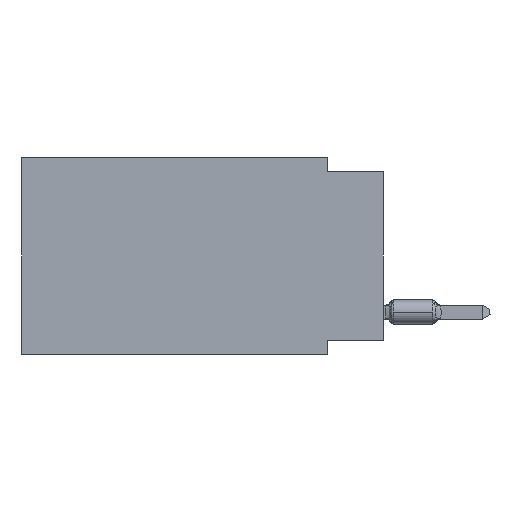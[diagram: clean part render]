
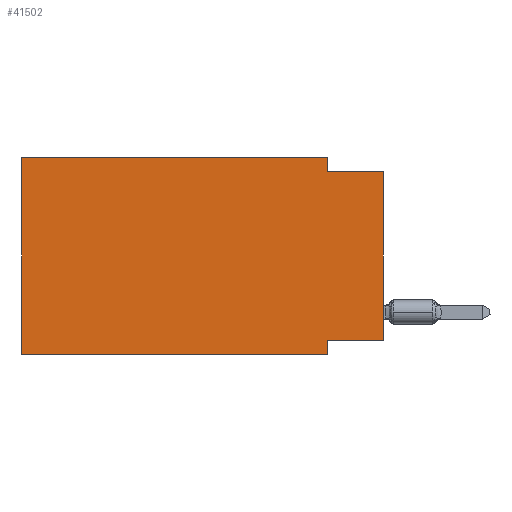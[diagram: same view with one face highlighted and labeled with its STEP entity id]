
A CAD part, left-side view. The second image highlights one B-rep face of the part: STEP entity #41502.
In plain terms, the highlighted planar face has unit normal (-1, 0, 0).
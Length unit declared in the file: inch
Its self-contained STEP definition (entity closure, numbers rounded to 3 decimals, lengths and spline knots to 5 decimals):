
#730 = LINE ( 'NONE', #33870, #26013 ) ;
#1937 = FACE_OUTER_BOUND ( 'NONE', #45939, .T. ) ;
#2708 = ORIENTED_EDGE ( 'NONE', *, *, #36477, .F. ) ;
#2786 = EDGE_CURVE ( 'NONE', #45251, #16510, #2845, .T. ) ;
#2845 = LINE ( 'NONE', #39812, #20690 ) ;
#5706 = DIRECTION ( 'NONE',  ( 0., 0., 1. ) ) ;
#6420 = LINE ( 'NONE', #46501, #44992 ) ;
#8974 = CARTESIAN_POINT ( 'NONE',  ( 0., 0.1, -0.35 ) ) ;
#9756 = ORIENTED_EDGE ( 'NONE', *, *, #10498, .T. ) ;
#9972 = DIRECTION ( 'NONE',  ( 0., -1., 0. ) ) ;
#10498 = EDGE_CURVE ( 'NONE', #33811, #16510, #16093, .T. ) ;
#12027 = DIRECTION ( 'NONE',  ( 0., 0., -1. ) ) ;
#12107 = CARTESIAN_POINT ( 'NONE',  ( 0., 0.645, 0. ) ) ;
#12514 = CARTESIAN_POINT ( 'NONE',  ( 0., 0.645, 0. ) ) ;
#13005 = LINE ( 'NONE', #16838, #44288 ) ;
#13292 = VECTOR ( 'NONE', #22812, 39.37008 ) ;
#15845 = DIRECTION ( 'NONE',  ( 0., -1., 0. ) ) ;
#16093 = LINE ( 'NONE', #41045, #37263 ) ;
#16480 = ORIENTED_EDGE ( 'NONE', *, *, #17004, .F. ) ;
#16510 = VERTEX_POINT ( 'NONE', #8974 ) ;
#16838 = CARTESIAN_POINT ( 'NONE',  ( 0., 0., -0.325 ) ) ;
#16841 = DIRECTION ( 'NONE',  ( 0., 0., -1. ) ) ;
#17004 = EDGE_CURVE ( 'NONE', #26796, #45251, #13005, .T. ) ;
#17196 = CARTESIAN_POINT ( 'NONE',  ( 0., 0., -0.025 ) ) ;
#17506 = DIRECTION ( 'NONE',  ( 0., 0., -1. ) ) ;
#18779 = EDGE_CURVE ( 'NONE', #23331, #19464, #730, .T. ) ;
#19195 = CARTESIAN_POINT ( 'NONE',  ( 0., 0.1, -0.325 ) ) ;
#19464 = VERTEX_POINT ( 'NONE', #34119 ) ;
#20690 = VECTOR ( 'NONE', #17506, 39.37008 ) ;
#20805 = CARTESIAN_POINT ( 'NONE',  ( 0., 0., -0.325 ) ) ;
#20972 = CARTESIAN_POINT ( 'NONE',  ( 0., 0.645, 0. ) ) ;
#21232 = VECTOR ( 'NONE', #26717, 39.37008 ) ;
#22812 = DIRECTION ( 'NONE',  ( 0., 0., 1. ) ) ;
#23331 = VERTEX_POINT ( 'NONE', #42076 ) ;
#23376 = LINE ( 'NONE', #12107, #21232 ) ;
#23537 = VECTOR ( 'NONE', #9972, 39.37008 ) ;
#24184 = EDGE_CURVE ( 'NONE', #26796, #29687, #6420, .T. ) ;
#26013 = VECTOR ( 'NONE', #12027, 39.37008 ) ;
#26717 = DIRECTION ( 'NONE',  ( 0., -1., 0. ) ) ;
#26796 = VERTEX_POINT ( 'NONE', #20805 ) ;
#29310 = VERTEX_POINT ( 'NONE', #20972 ) ;
#29471 = CARTESIAN_POINT ( 'NONE',  ( 0., 0., -0.025 ) ) ;
#29687 = VERTEX_POINT ( 'NONE', #29471 ) ;
#31001 = DIRECTION ( 'NONE',  ( 1., 0., 0. ) ) ;
#31341 = LINE ( 'NONE', #17196, #23537 ) ;
#31789 = ORIENTED_EDGE ( 'NONE', *, *, #2786, .F. ) ;
#32636 = ORIENTED_EDGE ( 'NONE', *, *, #24184, .T. ) ;
#33811 = VERTEX_POINT ( 'NONE', #34371 ) ;
#33870 = CARTESIAN_POINT ( 'NONE',  ( 0., 0.1, 0. ) ) ;
#33872 = LINE ( 'NONE', #12514, #13292 ) ;
#34119 = CARTESIAN_POINT ( 'NONE',  ( 0., 0.1, -0.025 ) ) ;
#34371 = CARTESIAN_POINT ( 'NONE',  ( 0., 0.645, -0.35 ) ) ;
#35066 = CARTESIAN_POINT ( 'NONE',  ( 0., 0.645, 0. ) ) ;
#36477 = EDGE_CURVE ( 'NONE', #33811, #29310, #33872, .T. ) ;
#37263 = VECTOR ( 'NONE', #15845, 39.37008 ) ;
#38706 = EDGE_CURVE ( 'NONE', #19464, #29687, #31341, .T. ) ;
#38974 = EDGE_CURVE ( 'NONE', #29310, #23331, #23376, .T. ) ;
#39812 = CARTESIAN_POINT ( 'NONE',  ( 0., 0.1, -0.35 ) ) ;
#41045 = CARTESIAN_POINT ( 'NONE',  ( 0., 0.645, -0.35 ) ) ;
#41502 = ADVANCED_FACE ( 'NONE', ( #1937 ), #41806, .F. ) ;
#41671 = ORIENTED_EDGE ( 'NONE', *, *, #38974, .F. ) ;
#41806 = PLANE ( 'NONE',  #43701 ) ;
#42076 = CARTESIAN_POINT ( 'NONE',  ( 0., 0.1, 0. ) ) ;
#42252 = ORIENTED_EDGE ( 'NONE', *, *, #38706, .F. ) ;
#43701 = AXIS2_PLACEMENT_3D ( 'NONE', #35066, #31001, #16841 ) ;
#44288 = VECTOR ( 'NONE', #45866, 39.37008 ) ;
#44992 = VECTOR ( 'NONE', #5706, 39.37008 ) ;
#45251 = VERTEX_POINT ( 'NONE', #19195 ) ;
#45866 = DIRECTION ( 'NONE',  ( 0., 1., 0. ) ) ;
#45939 = EDGE_LOOP ( 'NONE', ( #32636, #42252, #46641, #41671, #2708, #9756, #31789, #16480 ) ) ;
#46501 = CARTESIAN_POINT ( 'NONE',  ( 0., 0., 0. ) ) ;
#46641 = ORIENTED_EDGE ( 'NONE', *, *, #18779, .F. ) ;
